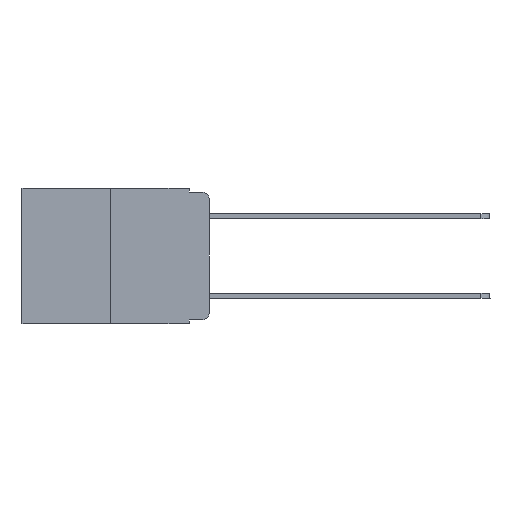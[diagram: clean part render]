
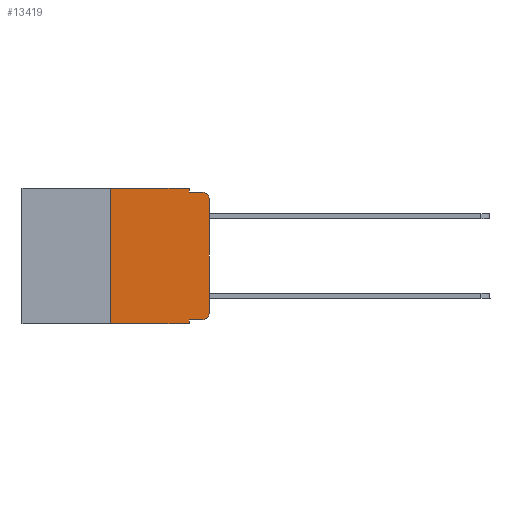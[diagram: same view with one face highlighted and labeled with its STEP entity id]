
A CAD part, left-side view. The second image highlights one B-rep face of the part: STEP entity #13419.
In plain terms, the highlighted planar face has unit normal (-1, 0, 0).
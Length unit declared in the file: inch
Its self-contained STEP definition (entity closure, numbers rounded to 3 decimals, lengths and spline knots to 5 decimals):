
#975 = CARTESIAN_POINT ( 'NONE',  ( 0., 0.473, 0. ) ) ;
#1102 = DIRECTION ( 'NONE',  ( 0., 0., 1. ) ) ;
#1135 = DIRECTION ( 'NONE',  ( -1., 0., 0. ) ) ;
#1448 = CARTESIAN_POINT ( 'NONE',  ( 0., 0.051, -0.343 ) ) ;
#1485 = LINE ( 'NONE', #3886, #8247 ) ;
#1563 = DIRECTION ( 'NONE',  ( 0., 0., -1. ) ) ;
#1598 = ORIENTED_EDGE ( 'NONE', *, *, #9077, .F. ) ;
#1669 = CARTESIAN_POINT ( 'NONE',  ( 0., 0.051, -0.01 ) ) ;
#1732 = DIRECTION ( 'NONE',  ( 0., 0., 1. ) ) ;
#1788 = EDGE_CURVE ( 'NONE', #5444, #6900, #5850, .T. ) ;
#2040 = DIRECTION ( 'NONE',  ( 0., 0., -1. ) ) ;
#2077 = CARTESIAN_POINT ( 'NONE',  ( 0., 0.02, -0.01 ) ) ;
#2086 = CARTESIAN_POINT ( 'NONE',  ( 0., 0.051, 0. ) ) ;
#2279 = CARTESIAN_POINT ( 'NONE',  ( 0., 0., -0.313 ) ) ;
#2371 = DIRECTION ( 'NONE',  ( 0., 0., -1. ) ) ;
#2513 = EDGE_CURVE ( 'NONE', #4699, #13698, #12336, .T. ) ;
#2541 = VECTOR ( 'NONE', #13652, 39.37008 ) ;
#2836 = CARTESIAN_POINT ( 'NONE',  ( 0., 0.051, -0.333 ) ) ;
#3127 = DIRECTION ( 'NONE',  ( 1., 0., 0. ) ) ;
#3886 = CARTESIAN_POINT ( 'NONE',  ( 0., 0.25, 0. ) ) ;
#4284 = EDGE_CURVE ( 'NONE', #5444, #13698, #9860, .T. ) ;
#4476 = VERTEX_POINT ( 'NONE', #5178 ) ;
#4620 = VECTOR ( 'NONE', #8748, 39.37008 ) ;
#4699 = VERTEX_POINT ( 'NONE', #6619 ) ;
#4824 = ORIENTED_EDGE ( 'NONE', *, *, #7606, .T. ) ;
#4931 = ORIENTED_EDGE ( 'NONE', *, *, #11637, .T. ) ;
#5075 = CARTESIAN_POINT ( 'NONE',  ( 0., 0.051, -0.01 ) ) ;
#5109 = FACE_OUTER_BOUND ( 'NONE', #12342, .T. ) ;
#5178 = CARTESIAN_POINT ( 'NONE',  ( 0., 0.25, 0. ) ) ;
#5277 = AXIS2_PLACEMENT_3D ( 'NONE', #8335, #13932, #1563 ) ;
#5444 = VERTEX_POINT ( 'NONE', #2836 ) ;
#5543 = ORIENTED_EDGE ( 'NONE', *, *, #1788, .T. ) ;
#5563 = CARTESIAN_POINT ( 'NONE',  ( 0., 0., -0.03 ) ) ;
#5735 = VERTEX_POINT ( 'NONE', #5563 ) ;
#5850 = LINE ( 'NONE', #13518, #2541 ) ;
#6008 = CIRCLE ( 'NONE', #10359, 0.02 ) ;
#6111 = CARTESIAN_POINT ( 'NONE',  ( 0., 0.02, -0.333 ) ) ;
#6338 = VERTEX_POINT ( 'NONE', #1669 ) ;
#6619 = CARTESIAN_POINT ( 'NONE',  ( 0., 0.25, -0.343 ) ) ;
#6726 = LINE ( 'NONE', #5075, #10020 ) ;
#6900 = VERTEX_POINT ( 'NONE', #6111 ) ;
#7406 = PLANE ( 'NONE',  #8913 ) ;
#7443 = VERTEX_POINT ( 'NONE', #8415 ) ;
#7547 = CARTESIAN_POINT ( 'NONE',  ( 0., 0.473, 0. ) ) ;
#7606 = EDGE_CURVE ( 'NONE', #10940, #5735, #11890, .T. ) ;
#8060 = ORIENTED_EDGE ( 'NONE', *, *, #10529, .F. ) ;
#8247 = VECTOR ( 'NONE', #1732, 39.37008 ) ;
#8335 = CARTESIAN_POINT ( 'NONE',  ( 0., 0.02, -0.313 ) ) ;
#8415 = CARTESIAN_POINT ( 'NONE',  ( 0., 0.051, 0. ) ) ;
#8489 = DIRECTION ( 'NONE',  ( 0., 0., -1. ) ) ;
#8748 = DIRECTION ( 'NONE',  ( 0., -1., 0. ) ) ;
#8913 = AXIS2_PLACEMENT_3D ( 'NONE', #7547, #3127, #2040 ) ;
#8941 = CARTESIAN_POINT ( 'NONE',  ( 0., 0.02, -0.03 ) ) ;
#8942 = DIRECTION ( 'NONE',  ( 0., -1., 0. ) ) ;
#9077 = EDGE_CURVE ( 'NONE', #7443, #6338, #12312, .T. ) ;
#9360 = VECTOR ( 'NONE', #8489, 39.37008 ) ;
#9382 = VECTOR ( 'NONE', #8942, 39.37008 ) ;
#9497 = DIRECTION ( 'NONE',  ( 0., -1., 0. ) ) ;
#9538 = ORIENTED_EDGE ( 'NONE', *, *, #11533, .F. ) ;
#9619 = ORIENTED_EDGE ( 'NONE', *, *, #12605, .F. ) ;
#9636 = ORIENTED_EDGE ( 'NONE', *, *, #4284, .F. ) ;
#9860 = LINE ( 'NONE', #2086, #11952 ) ;
#9914 = VERTEX_POINT ( 'NONE', #2077 ) ;
#9998 = CARTESIAN_POINT ( 'NONE',  ( 0., 0., 0. ) ) ;
#10020 = VECTOR ( 'NONE', #9497, 39.37008 ) ;
#10159 = ORIENTED_EDGE ( 'NONE', *, *, #11865, .T. ) ;
#10166 = CIRCLE ( 'NONE', #5277, 0.02 ) ;
#10359 = AXIS2_PLACEMENT_3D ( 'NONE', #8941, #1135, #2371 ) ;
#10529 = EDGE_CURVE ( 'NONE', #6338, #9914, #6726, .T. ) ;
#10940 = VERTEX_POINT ( 'NONE', #2279 ) ;
#11132 = CARTESIAN_POINT ( 'NONE',  ( 0., 0.473, -0.343 ) ) ;
#11186 = ORIENTED_EDGE ( 'NONE', *, *, #2513, .T. ) ;
#11533 = EDGE_CURVE ( 'NONE', #4476, #7443, #14142, .T. ) ;
#11614 = CARTESIAN_POINT ( 'NONE',  ( 0., 0.051, 0. ) ) ;
#11637 = EDGE_CURVE ( 'NONE', #5735, #9914, #6008, .T. ) ;
#11701 = VECTOR ( 'NONE', #1102, 39.37008 ) ;
#11865 = EDGE_CURVE ( 'NONE', #6900, #10940, #10166, .T. ) ;
#11890 = LINE ( 'NONE', #9998, #11701 ) ;
#11952 = VECTOR ( 'NONE', #14232, 39.37008 ) ;
#12312 = LINE ( 'NONE', #11614, #9360 ) ;
#12336 = LINE ( 'NONE', #11132, #9382 ) ;
#12342 = EDGE_LOOP ( 'NONE', ( #4824, #4931, #8060, #1598, #9538, #9619, #11186, #9636, #5543, #10159 ) ) ;
#12605 = EDGE_CURVE ( 'NONE', #4699, #4476, #1485, .T. ) ;
#13419 = ADVANCED_FACE ( 'NONE', ( #5109 ), #7406, .F. ) ;
#13518 = CARTESIAN_POINT ( 'NONE',  ( 0., 0.051, -0.333 ) ) ;
#13652 = DIRECTION ( 'NONE',  ( 0., -1., 0. ) ) ;
#13698 = VERTEX_POINT ( 'NONE', #1448 ) ;
#13932 = DIRECTION ( 'NONE',  ( -1., 0., 0. ) ) ;
#14142 = LINE ( 'NONE', #975, #4620 ) ;
#14232 = DIRECTION ( 'NONE',  ( 0., 0., -1. ) ) ;
